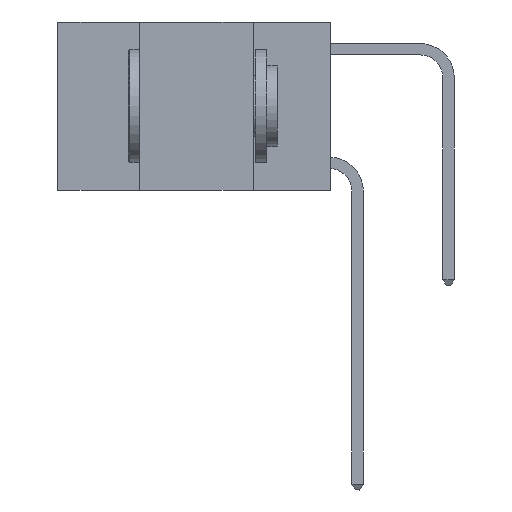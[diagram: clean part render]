
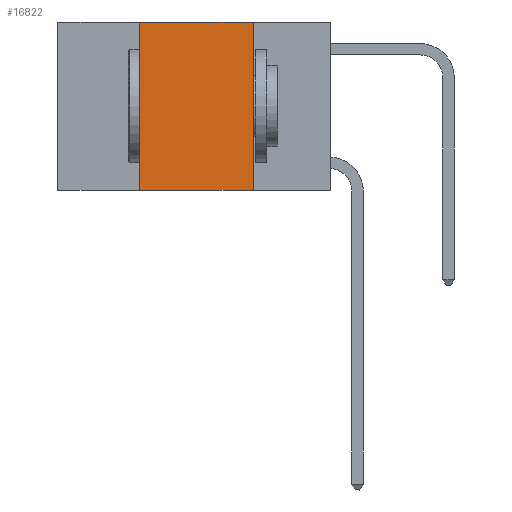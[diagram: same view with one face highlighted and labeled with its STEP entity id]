
A CAD part, left-side view. The second image highlights one B-rep face of the part: STEP entity #16822.
In plain terms, the highlighted planar face has unit normal (-1, 0, 0).
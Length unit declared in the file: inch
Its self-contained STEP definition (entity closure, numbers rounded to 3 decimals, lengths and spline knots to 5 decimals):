
#3338 = VECTOR ( 'NONE', #14196, 39.37008 ) ;
#3355 = VERTEX_POINT ( 'NONE', #12667 ) ;
#4033 = ORIENTED_EDGE ( 'NONE', *, *, #29370, .F. ) ;
#4041 = LINE ( 'NONE', #14564, #13960 ) ;
#4224 = EDGE_LOOP ( 'NONE', ( #4033, #29834, #5075, #31273 ) ) ;
#4711 = EDGE_CURVE ( 'NONE', #23349, #3355, #11057, .T. ) ;
#5075 = ORIENTED_EDGE ( 'NONE', *, *, #4711, .F. ) ;
#6288 = VERTEX_POINT ( 'NONE', #13801 ) ;
#8520 = DIRECTION ( 'NONE',  ( 1., 0., 0. ) ) ;
#8557 = LINE ( 'NONE', #19282, #3338 ) ;
#8953 = EDGE_CURVE ( 'NONE', #3355, #6288, #32076, .T. ) ;
#10651 = AXIS2_PLACEMENT_3D ( 'NONE', #33064, #8520, #22209 ) ;
#11057 = LINE ( 'NONE', #30372, #23008 ) ;
#12667 = CARTESIAN_POINT ( 'NONE',  ( 0., 0.42, 0. ) ) ;
#13801 = CARTESIAN_POINT ( 'NONE',  ( 0., 0.17, 0. ) ) ;
#13960 = VECTOR ( 'NONE', #27348, 39.37008 ) ;
#14196 = DIRECTION ( 'NONE',  ( 0., 0., -1. ) ) ;
#14564 = CARTESIAN_POINT ( 'NONE',  ( 0., 0.6, -0.37 ) ) ;
#14701 = PLANE ( 'NONE',  #10651 ) ;
#16763 = VECTOR ( 'NONE', #23869, 39.37008 ) ;
#16822 = ADVANCED_FACE ( 'NONE', ( #19957 ), #14701, .F. ) ;
#19152 = DIRECTION ( 'NONE',  ( 0., 0., 1. ) ) ;
#19282 = CARTESIAN_POINT ( 'NONE',  ( 0., 0.17, 0. ) ) ;
#19957 = FACE_OUTER_BOUND ( 'NONE', #4224, .T. ) ;
#20794 = CARTESIAN_POINT ( 'NONE',  ( 0., 0.17, -0.37 ) ) ;
#21928 = CARTESIAN_POINT ( 'NONE',  ( 0., 0.6, 0. ) ) ;
#22209 = DIRECTION ( 'NONE',  ( 0., 0., -1. ) ) ;
#23008 = VECTOR ( 'NONE', #19152, 39.37008 ) ;
#23306 = CARTESIAN_POINT ( 'NONE',  ( 0., 0.42, -0.37 ) ) ;
#23349 = VERTEX_POINT ( 'NONE', #23306 ) ;
#23869 = DIRECTION ( 'NONE',  ( 0., -1., 0. ) ) ;
#26434 = VERTEX_POINT ( 'NONE', #20794 ) ;
#27348 = DIRECTION ( 'NONE',  ( 0., -1., 0. ) ) ;
#29293 = EDGE_CURVE ( 'NONE', #23349, #26434, #4041, .T. ) ;
#29370 = EDGE_CURVE ( 'NONE', #6288, #26434, #8557, .T. ) ;
#29834 = ORIENTED_EDGE ( 'NONE', *, *, #8953, .F. ) ;
#30372 = CARTESIAN_POINT ( 'NONE',  ( 0., 0.42, 0. ) ) ;
#31273 = ORIENTED_EDGE ( 'NONE', *, *, #29293, .T. ) ;
#32076 = LINE ( 'NONE', #21928, #16763 ) ;
#33064 = CARTESIAN_POINT ( 'NONE',  ( 0., 0.6, 0. ) ) ;
